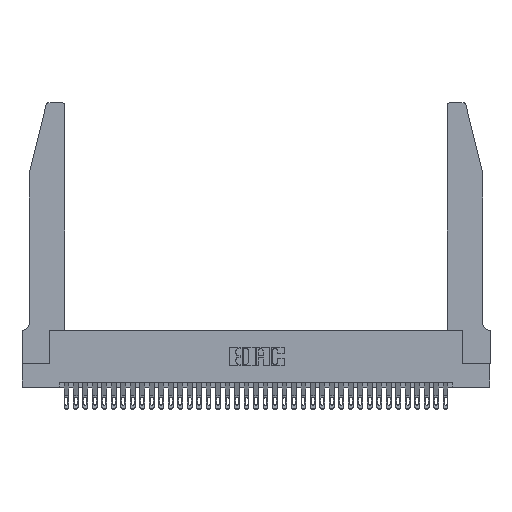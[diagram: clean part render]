
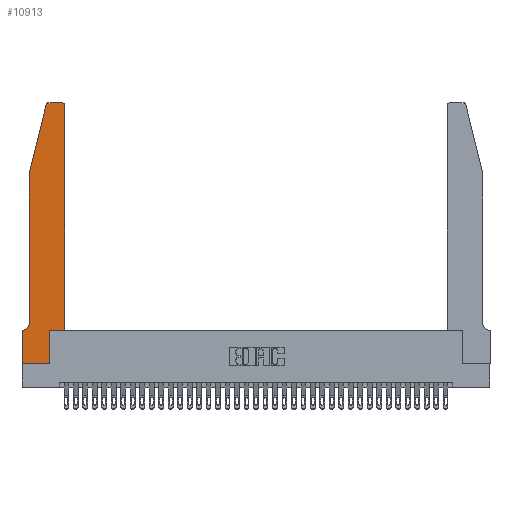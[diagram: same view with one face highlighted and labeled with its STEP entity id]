
A CAD part, top view. The second image highlights one B-rep face of the part: STEP entity #10913.
In plain terms, the highlighted planar face has unit normal (0, 0, 1).
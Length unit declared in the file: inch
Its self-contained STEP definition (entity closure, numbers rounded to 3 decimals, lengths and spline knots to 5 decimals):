
#335 = DIRECTION ( 'NONE',  ( 0., 1., 0. ) ) ;
#541 = VERTEX_POINT ( 'NONE', #34049 ) ;
#864 = ORIENTED_EDGE ( 'NONE', *, *, #15519, .T. ) ;
#1202 = VECTOR ( 'NONE', #34526, 39.37008 ) ;
#1391 = CARTESIAN_POINT ( 'NONE',  ( 0.4505, 0.35, 0.37 ) ) ;
#1502 = VECTOR ( 'NONE', #17004, 39.37008 ) ;
#1834 = CARTESIAN_POINT ( 'NONE',  ( 0.0755, 0.42, 0.37 ) ) ;
#1848 = DIRECTION ( 'NONE',  ( -1., 0., 0. ) ) ;
#2139 = CARTESIAN_POINT ( 'NONE',  ( 0.0755, 0.35, 0.37 ) ) ;
#2402 = LINE ( 'NONE', #2139, #9316 ) ;
#2991 = VERTEX_POINT ( 'NONE', #27179 ) ;
#3143 = ORIENTED_EDGE ( 'NONE', *, *, #3700, .T. ) ;
#3221 = DIRECTION ( 'NONE',  ( 0., 0., 1. ) ) ;
#3500 = DIRECTION ( 'NONE',  ( 0., 0., 1. ) ) ;
#3700 = EDGE_CURVE ( 'NONE', #18121, #15194, #6382, .T. ) ;
#5465 = VECTOR ( 'NONE', #36450, 39.37008 ) ;
#5769 = DIRECTION ( 'NONE',  ( 0., 1., 0. ) ) ;
#6382 = LINE ( 'NONE', #27876, #5465 ) ;
#6686 = EDGE_CURVE ( 'NONE', #2991, #11741, #35767, .T. ) ;
#6739 = EDGE_CURVE ( 'NONE', #14010, #29541, #2402, .T. ) ;
#6940 = CARTESIAN_POINT ( 'NONE',  ( 0.25487, 2.72718, 0.37 ) ) ;
#7167 = CARTESIAN_POINT ( 'NONE',  ( 0.0055, 0.35, 0.37 ) ) ;
#7766 = VECTOR ( 'NONE', #31868, 39.37008 ) ;
#7831 = LINE ( 'NONE', #27940, #29865 ) ;
#7890 = ORIENTED_EDGE ( 'NONE', *, *, #12040, .T. ) ;
#8467 = EDGE_CURVE ( 'NONE', #25513, #2991, #7831, .T. ) ;
#8673 = CARTESIAN_POINT ( 'NONE',  ( 0.4505, 0.35, 0.37 ) ) ;
#8937 = VERTEX_POINT ( 'NONE', #12647 ) ;
#9255 = VECTOR ( 'NONE', #10173, 39.37008 ) ;
#9316 = VECTOR ( 'NONE', #25336, 39.37008 ) ;
#9390 = EDGE_CURVE ( 'NONE', #11741, #23119, #30700, .T. ) ;
#9992 = LINE ( 'NONE', #28827, #1202 ) ;
#10173 = DIRECTION ( 'NONE',  ( 1., 0., 0. ) ) ;
#10913 = ADVANCED_FACE ( 'NONE', ( #18451 ), #20876, .T. ) ;
#11741 = VERTEX_POINT ( 'NONE', #6940 ) ;
#12040 = EDGE_CURVE ( 'NONE', #23119, #14182, #18812, .T. ) ;
#12195 = EDGE_LOOP ( 'NONE', ( #22782, #28921, #31840, #7890, #16559, #23443, #16263, #3143, #864, #15951, #25438, #20660 ) ) ;
#12508 = AXIS2_PLACEMENT_3D ( 'NONE', #29410, #3500, #23765 ) ;
#12591 = CARTESIAN_POINT ( 'NONE',  ( 0.2865, 0., 0.37 ) ) ;
#12647 = CARTESIAN_POINT ( 'NONE',  ( 0.2865, 0.35, 0.37 ) ) ;
#12660 = CARTESIAN_POINT ( 'NONE',  ( 0., 0., 0.37 ) ) ;
#12880 = AXIS2_PLACEMENT_3D ( 'NONE', #33375, #16197, #36240 ) ;
#14010 = VERTEX_POINT ( 'NONE', #7167 ) ;
#14086 = CARTESIAN_POINT ( 'NONE',  ( 0.0755, 2., 0.37 ) ) ;
#14182 = VERTEX_POINT ( 'NONE', #1834 ) ;
#15194 = VERTEX_POINT ( 'NONE', #12591 ) ;
#15519 = EDGE_CURVE ( 'NONE', #15194, #8937, #28102, .T. ) ;
#15951 = ORIENTED_EDGE ( 'NONE', *, *, #31391, .T. ) ;
#16197 = DIRECTION ( 'NONE',  ( 0., 0., -1. ) ) ;
#16263 = ORIENTED_EDGE ( 'NONE', *, *, #20400, .T. ) ;
#16377 = CARTESIAN_POINT ( 'NONE',  ( 0.284, 2.72, 0.37 ) ) ;
#16559 = ORIENTED_EDGE ( 'NONE', *, *, #18294, .T. ) ;
#17004 = DIRECTION ( 'NONE',  ( 0., -1., 0. ) ) ;
#18020 = CARTESIAN_POINT ( 'NONE',  ( 0., 0.35, 0.37 ) ) ;
#18121 = VERTEX_POINT ( 'NONE', #12660 ) ;
#18294 = EDGE_CURVE ( 'NONE', #14182, #14010, #27510, .T. ) ;
#18451 = FACE_OUTER_BOUND ( 'NONE', #12195, .T. ) ;
#18633 = EDGE_CURVE ( 'NONE', #27213, #541, #25237, .T. ) ;
#18812 = LINE ( 'NONE', #14086, #1502 ) ;
#19292 = DIRECTION ( 'NONE',  ( 1., 0., 0. ) ) ;
#20267 = CIRCLE ( 'NONE', #24563, 0.03 ) ;
#20400 = EDGE_CURVE ( 'NONE', #29541, #18121, #9992, .T. ) ;
#20606 = CARTESIAN_POINT ( 'NONE',  ( 0.4205, 2.72, 0.37 ) ) ;
#20660 = ORIENTED_EDGE ( 'NONE', *, *, #21184, .T. ) ;
#20876 = PLANE ( 'NONE',  #12508 ) ;
#21184 = EDGE_CURVE ( 'NONE', #541, #25513, #20267, .T. ) ;
#22782 = ORIENTED_EDGE ( 'NONE', *, *, #8467, .T. ) ;
#23119 = VERTEX_POINT ( 'NONE', #35255 ) ;
#23381 = CARTESIAN_POINT ( 'NONE',  ( 0.0755, 2., 0.37 ) ) ;
#23443 = ORIENTED_EDGE ( 'NONE', *, *, #6739, .T. ) ;
#23501 = DIRECTION ( 'NONE',  ( 1., 0., 0. ) ) ;
#23765 = DIRECTION ( 'NONE',  ( 1., 0., 0. ) ) ;
#24563 = AXIS2_PLACEMENT_3D ( 'NONE', #20606, #3221, #23501 ) ;
#25237 = LINE ( 'NONE', #8673, #31935 ) ;
#25336 = DIRECTION ( 'NONE',  ( -1., 0., 0. ) ) ;
#25438 = ORIENTED_EDGE ( 'NONE', *, *, #18633, .T. ) ;
#25463 = LINE ( 'NONE', #1391, #9255 ) ;
#25513 = VERTEX_POINT ( 'NONE', #29180 ) ;
#25947 = CARTESIAN_POINT ( 'NONE',  ( 0.2865, 0.35, 0.37 ) ) ;
#27179 = CARTESIAN_POINT ( 'NONE',  ( 0.284, 2.75, 0.37 ) ) ;
#27213 = VERTEX_POINT ( 'NONE', #33653 ) ;
#27510 = CIRCLE ( 'NONE', #12880, 0.07 ) ;
#27876 = CARTESIAN_POINT ( 'NONE',  ( 0., 0., 0.37 ) ) ;
#27940 = CARTESIAN_POINT ( 'NONE',  ( 0.2605, 2.75, 0.37 ) ) ;
#28102 = LINE ( 'NONE', #25947, #36549 ) ;
#28827 = CARTESIAN_POINT ( 'NONE',  ( 0., 0., 0.37 ) ) ;
#28921 = ORIENTED_EDGE ( 'NONE', *, *, #6686, .T. ) ;
#29180 = CARTESIAN_POINT ( 'NONE',  ( 0.4205, 2.75, 0.37 ) ) ;
#29410 = CARTESIAN_POINT ( 'NONE',  ( 0., 0.35, 0.37 ) ) ;
#29541 = VERTEX_POINT ( 'NONE', #18020 ) ;
#29865 = VECTOR ( 'NONE', #1848, 39.37008 ) ;
#30700 = LINE ( 'NONE', #23381, #7766 ) ;
#31391 = EDGE_CURVE ( 'NONE', #8937, #27213, #25463, .T. ) ;
#31840 = ORIENTED_EDGE ( 'NONE', *, *, #9390, .T. ) ;
#31868 = DIRECTION ( 'NONE',  ( -0.239, -0.971, 0. ) ) ;
#31935 = VECTOR ( 'NONE', #335, 39.37008 ) ;
#33375 = CARTESIAN_POINT ( 'NONE',  ( 0.0055, 0.42, 0.37 ) ) ;
#33653 = CARTESIAN_POINT ( 'NONE',  ( 0.4505, 0.35, 0.37 ) ) ;
#34049 = CARTESIAN_POINT ( 'NONE',  ( 0.4505, 2.72, 0.37 ) ) ;
#34526 = DIRECTION ( 'NONE',  ( 0., -1., 0. ) ) ;
#34751 = AXIS2_PLACEMENT_3D ( 'NONE', #16377, #36415, #19292 ) ;
#35255 = CARTESIAN_POINT ( 'NONE',  ( 0.0755, 2., 0.37 ) ) ;
#35767 = CIRCLE ( 'NONE', #34751, 0.03 ) ;
#36240 = DIRECTION ( 'NONE',  ( -1., 0., 0. ) ) ;
#36415 = DIRECTION ( 'NONE',  ( 0., 0., 1. ) ) ;
#36450 = DIRECTION ( 'NONE',  ( 1., 0., 0. ) ) ;
#36549 = VECTOR ( 'NONE', #5769, 39.37008 ) ;
